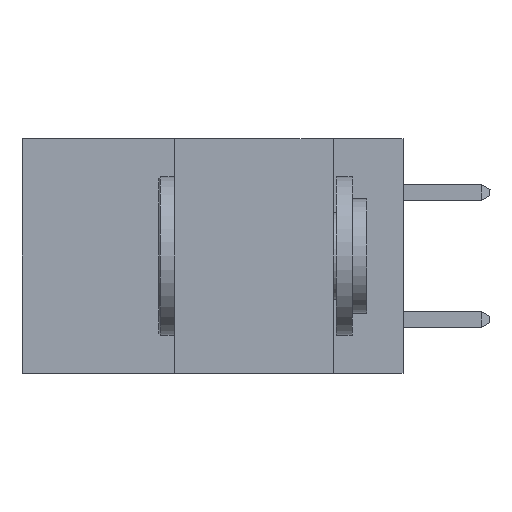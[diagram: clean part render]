
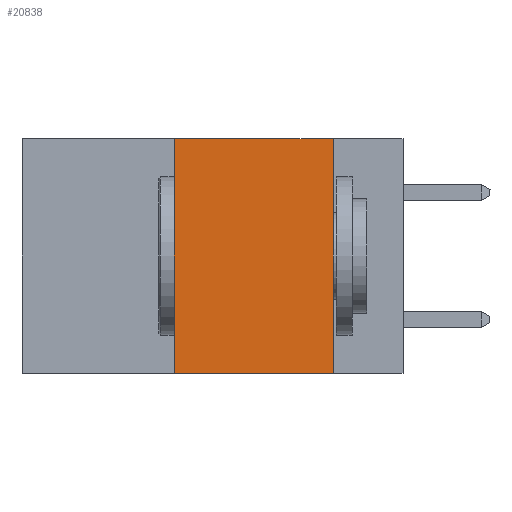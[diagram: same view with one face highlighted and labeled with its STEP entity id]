
A CAD part, left-side view. The second image highlights one B-rep face of the part: STEP entity #20838.
In plain terms, the highlighted planar face has unit normal (-1, 0, 0).
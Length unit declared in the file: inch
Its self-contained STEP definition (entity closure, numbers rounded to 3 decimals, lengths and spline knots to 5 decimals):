
#954 = PLANE ( 'NONE',  #15258 ) ;
#1074 = DIRECTION ( 'NONE',  ( 0., -1., 0. ) ) ;
#1675 = CARTESIAN_POINT ( 'NONE',  ( 0., 0.11, 0. ) ) ;
#2001 = VERTEX_POINT ( 'NONE', #26804 ) ;
#2543 = VECTOR ( 'NONE', #19369, 39.37008 ) ;
#3246 = LINE ( 'NONE', #25323, #10134 ) ;
#3292 = DIRECTION ( 'NONE',  ( 1., 0., 0. ) ) ;
#7681 = ORIENTED_EDGE ( 'NONE', *, *, #8658, .F. ) ;
#8658 = EDGE_CURVE ( 'NONE', #2001, #12064, #18140, .T. ) ;
#8717 = LINE ( 'NONE', #12393, #2543 ) ;
#10134 = VECTOR ( 'NONE', #11547, 39.37008 ) ;
#10176 = ORIENTED_EDGE ( 'NONE', *, *, #18949, .T. ) ;
#10621 = EDGE_CURVE ( 'NONE', #22918, #2001, #3246, .T. ) ;
#11547 = DIRECTION ( 'NONE',  ( 0., 0., 1. ) ) ;
#12064 = VERTEX_POINT ( 'NONE', #18615 ) ;
#12393 = CARTESIAN_POINT ( 'NONE',  ( 0., 0.6, -0.37 ) ) ;
#12720 = VECTOR ( 'NONE', #1074, 39.37008 ) ;
#13113 = VECTOR ( 'NONE', #15539, 39.37008 ) ;
#13201 = EDGE_LOOP ( 'NONE', ( #28106, #7681, #16713, #10176 ) ) ;
#14307 = VERTEX_POINT ( 'NONE', #24518 ) ;
#14927 = CARTESIAN_POINT ( 'NONE',  ( 0., 0.6, 0. ) ) ;
#15258 = AXIS2_PLACEMENT_3D ( 'NONE', #17142, #3292, #19478 ) ;
#15539 = DIRECTION ( 'NONE',  ( 0., 0., -1. ) ) ;
#16713 = ORIENTED_EDGE ( 'NONE', *, *, #10621, .F. ) ;
#17142 = CARTESIAN_POINT ( 'NONE',  ( 0., 0.6, 0. ) ) ;
#18140 = LINE ( 'NONE', #14927, #12720 ) ;
#18615 = CARTESIAN_POINT ( 'NONE',  ( 0., 0.11, 0. ) ) ;
#18949 = EDGE_CURVE ( 'NONE', #22918, #14307, #8717, .T. ) ;
#19369 = DIRECTION ( 'NONE',  ( 0., -1., 0. ) ) ;
#19478 = DIRECTION ( 'NONE',  ( 0., 0., -1. ) ) ;
#20838 = ADVANCED_FACE ( 'NONE', ( #29436 ), #954, .F. ) ;
#22918 = VERTEX_POINT ( 'NONE', #26660 ) ;
#24518 = CARTESIAN_POINT ( 'NONE',  ( 0., 0.11, -0.37 ) ) ;
#25323 = CARTESIAN_POINT ( 'NONE',  ( 0., 0.36, 0. ) ) ;
#25366 = LINE ( 'NONE', #1675, #13113 ) ;
#26039 = EDGE_CURVE ( 'NONE', #12064, #14307, #25366, .T. ) ;
#26660 = CARTESIAN_POINT ( 'NONE',  ( 0., 0.36, -0.37 ) ) ;
#26804 = CARTESIAN_POINT ( 'NONE',  ( 0., 0.36, 0. ) ) ;
#28106 = ORIENTED_EDGE ( 'NONE', *, *, #26039, .F. ) ;
#29436 = FACE_OUTER_BOUND ( 'NONE', #13201, .T. ) ;
